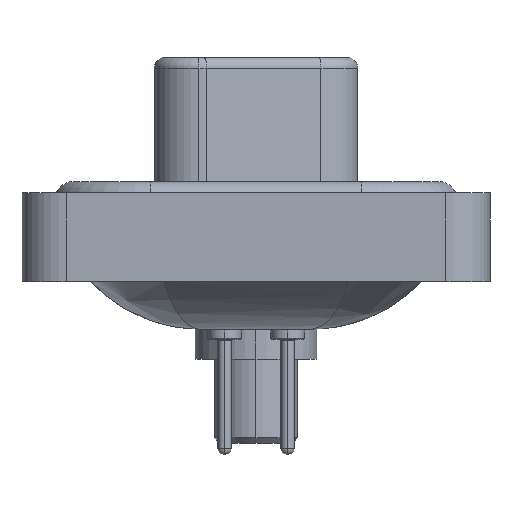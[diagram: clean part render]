
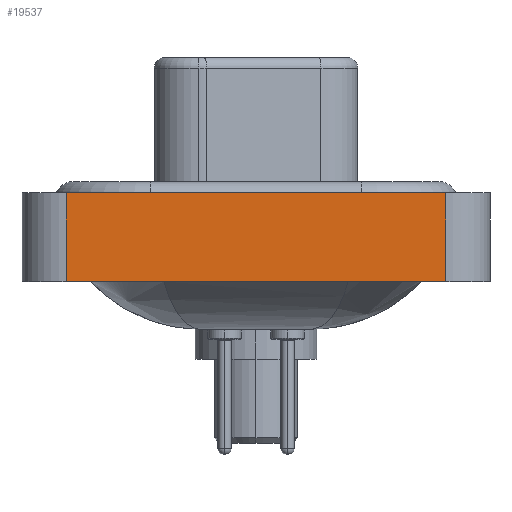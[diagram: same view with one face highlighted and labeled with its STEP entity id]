
A CAD part, left-side view. The second image highlights one B-rep face of the part: STEP entity #19537.
In plain terms, the highlighted planar face has unit normal (-1, 0, 0).
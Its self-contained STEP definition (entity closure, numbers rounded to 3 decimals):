
#325 = EDGE_CURVE ( 'NONE', #14824, #19782, #4708, .T. ) ;
#756 = CARTESIAN_POINT ( 'NONE',  ( -7.3, -8.55, 0.4 ) ) ;
#2395 = AXIS2_PLACEMENT_3D ( 'NONE', #17246, #20558, #4803 ) ;
#2663 = ORIENTED_EDGE ( 'NONE', *, *, #15557, .F. ) ;
#3020 = FACE_OUTER_BOUND ( 'NONE', #20202, .T. ) ;
#4708 = LINE ( 'NONE', #18049, #14446 ) ;
#4803 = DIRECTION ( 'NONE',  ( 0., 0., 1. ) ) ;
#4996 = VERTEX_POINT ( 'NONE', #8135 ) ;
#5619 = EDGE_CURVE ( 'NONE', #8042, #19782, #14555, .T. ) ;
#6325 = EDGE_CURVE ( 'NONE', #4996, #14824, #8762, .T. ) ;
#7184 = CARTESIAN_POINT ( 'NONE',  ( -7.3, 8.55, -3.6 ) ) ;
#7190 = ORIENTED_EDGE ( 'NONE', *, *, #5619, .F. ) ;
#8042 = VERTEX_POINT ( 'NONE', #11529 ) ;
#8135 = CARTESIAN_POINT ( 'NONE',  ( -7.3, 8.55, -3.6 ) ) ;
#8762 = LINE ( 'NONE', #13568, #9943 ) ;
#9512 = PLANE ( 'NONE',  #2395 ) ;
#9943 = VECTOR ( 'NONE', #15152, 1000. ) ;
#10418 = VECTOR ( 'NONE', #13250, 1000. ) ;
#10552 = ORIENTED_EDGE ( 'NONE', *, *, #6325, .T. ) ;
#10694 = CARTESIAN_POINT ( 'NONE',  ( -7.3, -8.55, -3.6 ) ) ;
#11099 = DIRECTION ( 'NONE',  ( 0., 0., 1. ) ) ;
#11529 = CARTESIAN_POINT ( 'NONE',  ( -7.3, 8.55, 0.4 ) ) ;
#13250 = DIRECTION ( 'NONE',  ( 0., 0., 1. ) ) ;
#13568 = CARTESIAN_POINT ( 'NONE',  ( -7.3, -8.55, -3.6 ) ) ;
#13591 = VECTOR ( 'NONE', #19534, 1000. ) ;
#14446 = VECTOR ( 'NONE', #11099, 1000. ) ;
#14555 = LINE ( 'NONE', #14865, #13591 ) ;
#14824 = VERTEX_POINT ( 'NONE', #10694 ) ;
#14865 = CARTESIAN_POINT ( 'NONE',  ( -7.3, -8.55, 0.4 ) ) ;
#15152 = DIRECTION ( 'NONE',  ( 0., -1., 0. ) ) ;
#15557 = EDGE_CURVE ( 'NONE', #4996, #8042, #18258, .T. ) ;
#17013 = ORIENTED_EDGE ( 'NONE', *, *, #325, .T. ) ;
#17246 = CARTESIAN_POINT ( 'NONE',  ( -7.3, -8.55, -3.6 ) ) ;
#18049 = CARTESIAN_POINT ( 'NONE',  ( -7.3, -8.55, -3.6 ) ) ;
#18258 = LINE ( 'NONE', #7184, #10418 ) ;
#19534 = DIRECTION ( 'NONE',  ( 0., -1., 0. ) ) ;
#19537 = ADVANCED_FACE ( 'NONE', ( #3020 ), #9512, .T. ) ;
#19782 = VERTEX_POINT ( 'NONE', #756 ) ;
#20202 = EDGE_LOOP ( 'NONE', ( #17013, #7190, #2663, #10552 ) ) ;
#20558 = DIRECTION ( 'NONE',  ( -1., 0., 0. ) ) ;
